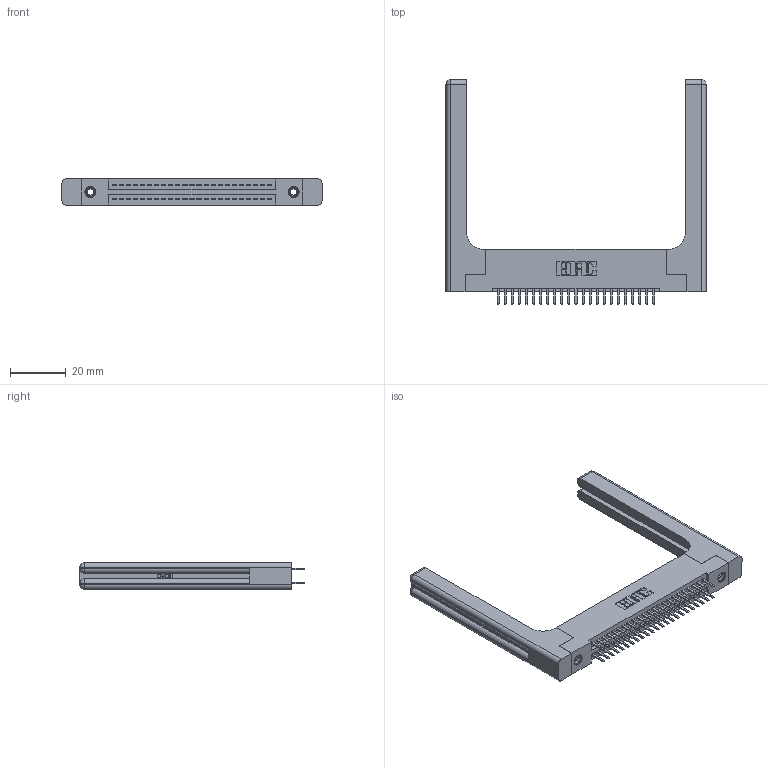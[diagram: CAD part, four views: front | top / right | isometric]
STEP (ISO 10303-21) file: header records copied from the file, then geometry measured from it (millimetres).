
FILE_DESCRIPTION (( 'STEP AP203' ), '1' );
FILE_NAME ('395-046-520-258.STEP', '2019-10-19T03:23:08', ( '' ), ( '' ), 'SwSTEP 2.0', 'SolidWorks 2016', '' );
FILE_SCHEMA (( 'CONFIG_CONTROL_DESIGN' ));
Length unit declared in the file: inch
Products named in the file (5): 345-250-001_345-250-001-102; 345-220-058_345-220-058; 395-046-520-258; 345 Part_Flush Mounting Lugs - 0.156 Dia-TH; 345-292-001_345-293-120
Assembly tree (51 placements, depth 2):
  395-046-520-258
    345 Part_Flush Mounting Lugs - 0.156 Dia-TH
    345-292-001_345-293-120  x46
    345-250-001_345-250-001-102  x2
    345-220-058_345-220-058  x2
Bounding box: 93.45 x 80.64 x 9.4 mm (x, y, z)
Volume: 17356 mm3; surface area: 17775.3 mm2
Topology: 51 solids, 51 shells, 2866 faces, 8229 edges, 5342 vertices
Faces by surface type: plane 1838, cylinder 968, bspline 36, cone 12, sphere 8, torus 4
Entity records: 25900 total; most frequent: CARTESIAN_POINT 5365, ORIENTED_EDGE 4084, DIRECTION 3674, EDGE_CURVE 2042, VECTOR 1722, LINE 1722, VERTEX_POINT 1350, AXIS2_PLACEMENT_3D 976
